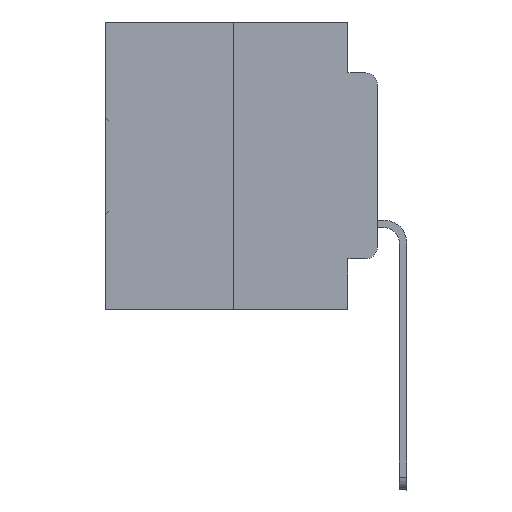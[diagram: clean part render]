
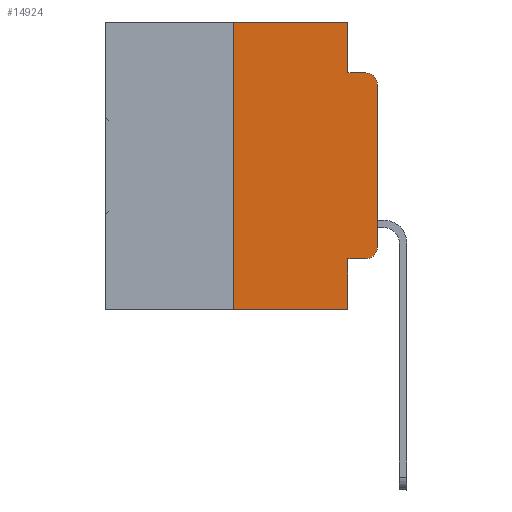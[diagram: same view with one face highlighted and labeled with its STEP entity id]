
A CAD part, left-side view. The second image highlights one B-rep face of the part: STEP entity #14924.
In plain terms, the highlighted planar face has unit normal (-1, 0, 0).
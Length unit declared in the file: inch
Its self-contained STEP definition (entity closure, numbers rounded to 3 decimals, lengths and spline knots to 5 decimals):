
#151 = AXIS2_PLACEMENT_3D ( 'NONE', #28764, #31532, #18740 ) ;
#240 = CARTESIAN_POINT ( 'NONE',  ( 0., 0., 0. ) ) ;
#411 = DIRECTION ( 'NONE',  ( 0., -1., 0. ) ) ;
#974 = VERTEX_POINT ( 'NONE', #2334 ) ;
#1269 = VERTEX_POINT ( 'NONE', #28768 ) ;
#1526 = VECTOR ( 'NONE', #28136, 39.37008 ) ;
#1793 = CARTESIAN_POINT ( 'NONE',  ( 0., 0.02, -0.3915 ) ) ;
#2028 = CARTESIAN_POINT ( 'NONE',  ( 0., 0.25, 0. ) ) ;
#2334 = CARTESIAN_POINT ( 'NONE',  ( 0., 0., -0.1085 ) ) ;
#2454 = DIRECTION ( 'NONE',  ( 0., -1., 0. ) ) ;
#2876 = CARTESIAN_POINT ( 'NONE',  ( 0., 0.473, -0.5 ) ) ;
#3175 = AXIS2_PLACEMENT_3D ( 'NONE', #1793, #29087, #11334 ) ;
#3864 = ORIENTED_EDGE ( 'NONE', *, *, #31386, .T. ) ;
#4352 = VECTOR ( 'NONE', #32414, 39.37008 ) ;
#4757 = VERTEX_POINT ( 'NONE', #24177 ) ;
#5390 = EDGE_CURVE ( 'NONE', #29822, #7694, #19856, .T. ) ;
#6056 = EDGE_CURVE ( 'NONE', #1269, #19336, #15376, .T. ) ;
#7201 = ORIENTED_EDGE ( 'NONE', *, *, #12913, .F. ) ;
#7469 = EDGE_CURVE ( 'NONE', #22140, #19336, #29006, .T. ) ;
#7694 = VERTEX_POINT ( 'NONE', #25526 ) ;
#8393 = FACE_OUTER_BOUND ( 'NONE', #10157, .T. ) ;
#8586 = CARTESIAN_POINT ( 'NONE',  ( 0., 0.02, -0.1085 ) ) ;
#9566 = EDGE_CURVE ( 'NONE', #19184, #28237, #20522, .T. ) ;
#9605 = LINE ( 'NONE', #2028, #4352 ) ;
#9671 = DIRECTION ( 'NONE',  ( 0., -1., 0. ) ) ;
#10157 = EDGE_LOOP ( 'NONE', ( #18976, #16914, #21772, #21830, #18864, #7201, #19026, #10278, #3864, #18280 ) ) ;
#10252 = DIRECTION ( 'NONE',  ( 0., 0., 1. ) ) ;
#10278 = ORIENTED_EDGE ( 'NONE', *, *, #7469, .F. ) ;
#10465 = EDGE_CURVE ( 'NONE', #4757, #974, #22759, .T. ) ;
#11012 = PLANE ( 'NONE',  #151 ) ;
#11334 = DIRECTION ( 'NONE',  ( 0., 0., -1. ) ) ;
#12331 = LINE ( 'NONE', #14793, #31472 ) ;
#12633 = DIRECTION ( 'NONE',  ( 0., -1., 0. ) ) ;
#12913 = EDGE_CURVE ( 'NONE', #1269, #29822, #9605, .T. ) ;
#13216 = VECTOR ( 'NONE', #10252, 39.37008 ) ;
#13336 = CARTESIAN_POINT ( 'NONE',  ( 0., 0.051, 0. ) ) ;
#13348 = DIRECTION ( 'NONE',  ( 0., 0., -1. ) ) ;
#13699 = VECTOR ( 'NONE', #12633, 39.37008 ) ;
#14793 = CARTESIAN_POINT ( 'NONE',  ( 0., 0.051, -0.4115 ) ) ;
#14924 = ADVANCED_FACE ( 'NONE', ( #8393 ), #11012, .F. ) ;
#15376 = LINE ( 'NONE', #2876, #22441 ) ;
#15684 = VERTEX_POINT ( 'NONE', #25394 ) ;
#16657 = CARTESIAN_POINT ( 'NONE',  ( 0., 0.051, 0. ) ) ;
#16914 = ORIENTED_EDGE ( 'NONE', *, *, #28233, .T. ) ;
#17563 = CARTESIAN_POINT ( 'NONE',  ( 0., 0.473, 0. ) ) ;
#18211 = VECTOR ( 'NONE', #9671, 39.37008 ) ;
#18280 = ORIENTED_EDGE ( 'NONE', *, *, #27430, .T. ) ;
#18740 = DIRECTION ( 'NONE',  ( 0., 0., -1. ) ) ;
#18864 = ORIENTED_EDGE ( 'NONE', *, *, #5390, .F. ) ;
#18892 = VECTOR ( 'NONE', #19135, 39.37008 ) ;
#18976 = ORIENTED_EDGE ( 'NONE', *, *, #10465, .T. ) ;
#19026 = ORIENTED_EDGE ( 'NONE', *, *, #6056, .T. ) ;
#19135 = DIRECTION ( 'NONE',  ( 0., 0., -1. ) ) ;
#19184 = VERTEX_POINT ( 'NONE', #22596 ) ;
#19336 = VERTEX_POINT ( 'NONE', #25556 ) ;
#19433 = CIRCLE ( 'NONE', #3175, 0.02 ) ;
#19856 = LINE ( 'NONE', #17563, #18211 ) ;
#20522 = LINE ( 'NONE', #30058, #13699 ) ;
#20576 = LINE ( 'NONE', #13336, #1526 ) ;
#20747 = DIRECTION ( 'NONE',  ( -1., 0., 0. ) ) ;
#20758 = CARTESIAN_POINT ( 'NONE',  ( 0., 0.051, -0.4115 ) ) ;
#21560 = CIRCLE ( 'NONE', #25781, 0.02 ) ;
#21772 = ORIENTED_EDGE ( 'NONE', *, *, #9566, .F. ) ;
#21830 = ORIENTED_EDGE ( 'NONE', *, *, #31149, .F. ) ;
#22140 = VERTEX_POINT ( 'NONE', #20758 ) ;
#22441 = VECTOR ( 'NONE', #411, 39.37008 ) ;
#22596 = CARTESIAN_POINT ( 'NONE',  ( 0., 0.051, -0.0885 ) ) ;
#22759 = LINE ( 'NONE', #240, #13216 ) ;
#24177 = CARTESIAN_POINT ( 'NONE',  ( 0., 0., -0.3915 ) ) ;
#25394 = CARTESIAN_POINT ( 'NONE',  ( 0., 0.02, -0.4115 ) ) ;
#25526 = CARTESIAN_POINT ( 'NONE',  ( 0., 0.051, 0. ) ) ;
#25556 = CARTESIAN_POINT ( 'NONE',  ( 0., 0.051, -0.5 ) ) ;
#25781 = AXIS2_PLACEMENT_3D ( 'NONE', #8586, #20747, #13348 ) ;
#26162 = CARTESIAN_POINT ( 'NONE',  ( 0., 0.02, -0.0885 ) ) ;
#27430 = EDGE_CURVE ( 'NONE', #15684, #4757, #19433, .T. ) ;
#28136 = DIRECTION ( 'NONE',  ( 0., 0., -1. ) ) ;
#28233 = EDGE_CURVE ( 'NONE', #974, #28237, #21560, .T. ) ;
#28237 = VERTEX_POINT ( 'NONE', #26162 ) ;
#28249 = CARTESIAN_POINT ( 'NONE',  ( 0., 0.25, 0. ) ) ;
#28764 = CARTESIAN_POINT ( 'NONE',  ( 0., 0.473, 0. ) ) ;
#28768 = CARTESIAN_POINT ( 'NONE',  ( 0., 0.25, -0.5 ) ) ;
#29006 = LINE ( 'NONE', #16657, #18892 ) ;
#29087 = DIRECTION ( 'NONE',  ( -1., 0., 0. ) ) ;
#29822 = VERTEX_POINT ( 'NONE', #28249 ) ;
#30058 = CARTESIAN_POINT ( 'NONE',  ( 0., 0.051, -0.0885 ) ) ;
#31149 = EDGE_CURVE ( 'NONE', #7694, #19184, #20576, .T. ) ;
#31386 = EDGE_CURVE ( 'NONE', #22140, #15684, #12331, .T. ) ;
#31472 = VECTOR ( 'NONE', #2454, 39.37008 ) ;
#31532 = DIRECTION ( 'NONE',  ( 1., 0., 0. ) ) ;
#32414 = DIRECTION ( 'NONE',  ( 0., 0., 1. ) ) ;
